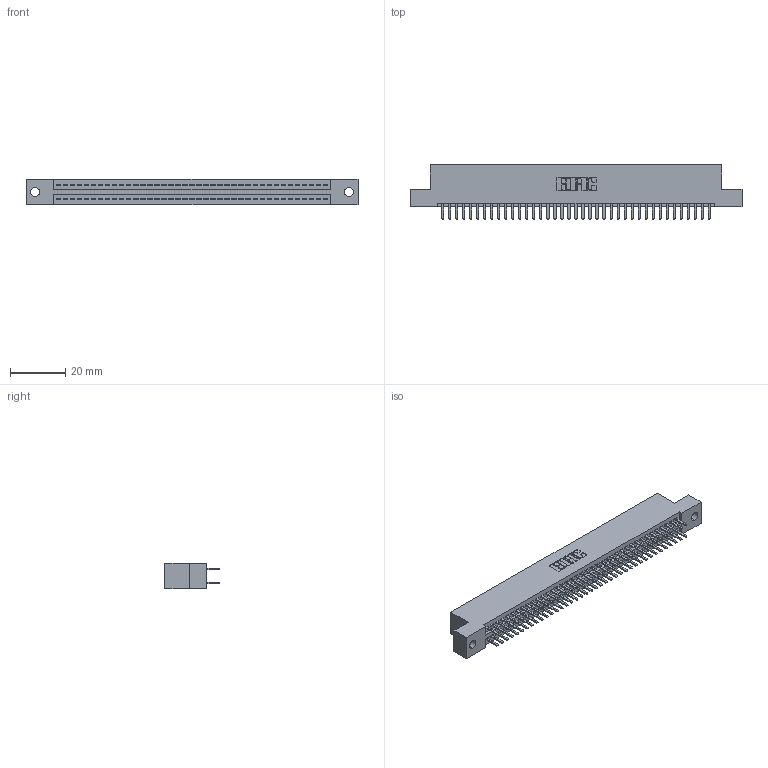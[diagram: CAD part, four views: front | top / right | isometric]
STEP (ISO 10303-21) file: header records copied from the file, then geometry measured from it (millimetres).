
FILE_DESCRIPTION (( 'STEP AP203' ), '1' );
FILE_NAME ('395-078-520-202.STEP', '2018-11-27T23:16:48', ( '' ), ( '' ), 'SwSTEP 2.0', 'SolidWorks 2016', '' );
FILE_SCHEMA (( 'CONFIG_CONTROL_DESIGN' ));
Length unit declared in the file: inch
Products named in the file (3): 395-078-520-202; 345-292-001_345-293-120; 345 Part_Flush Mounting Lugs - 0.128 Dia
Assembly tree (79 placements, depth 2):
  395-078-520-202
    345 Part_Flush Mounting Lugs - 0.128 Dia
    345-292-001_345-293-120  x78
Bounding box: 120.27 x 19.68 x 9.4 mm (x, y, z)
Volume: 11584.2 mm3; surface area: 16719.7 mm2
Topology: 79 solids, 79 shells, 4338 faces, 12587 edges, 8182 vertices
Faces by surface type: plane 2810, cylinder 1528
Entity records: 31121 total; most frequent: CARTESIAN_POINT 5232, ORIENTED_EDGE 5154, DIRECTION 4605, EDGE_CURVE 2577, LINE 2285, VECTOR 2285, VERTEX_POINT 1714, AXIS2_PLACEMENT_3D 1160
